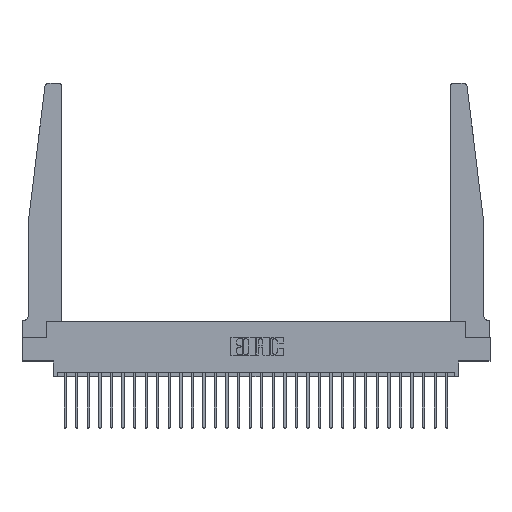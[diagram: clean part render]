
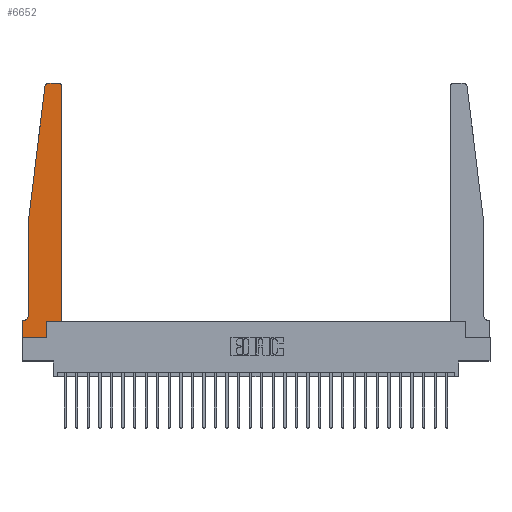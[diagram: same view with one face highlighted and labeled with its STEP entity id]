
A CAD part, top view. The second image highlights one B-rep face of the part: STEP entity #6652.
In plain terms, the highlighted planar face has unit normal (0, 0, 1).
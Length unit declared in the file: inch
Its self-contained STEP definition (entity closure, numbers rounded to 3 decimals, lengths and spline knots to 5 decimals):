
#420 = DIRECTION ( 'NONE',  ( -1., 0., 0. ) ) ;
#589 = ORIENTED_EDGE ( 'NONE', *, *, #18450, .T. ) ;
#660 = ORIENTED_EDGE ( 'NONE', *, *, #11698, .T. ) ;
#1101 = CARTESIAN_POINT ( 'NONE',  ( 0.065, 1.25, 0.37 ) ) ;
#1599 = VECTOR ( 'NONE', #24803, 39.37008 ) ;
#1626 = DIRECTION ( 'NONE',  ( 1., 0., 0. ) ) ;
#1912 = VECTOR ( 'NONE', #25168, 39.37008 ) ;
#2360 = CARTESIAN_POINT ( 'NONE',  ( 0.425, 2.72, 0.37 ) ) ;
#3061 = VECTOR ( 'NONE', #420, 39.37008 ) ;
#3380 = VERTEX_POINT ( 'NONE', #21767 ) ;
#3493 = VERTEX_POINT ( 'NONE', #7417 ) ;
#3578 = DIRECTION ( 'NONE',  ( 0., -1., 0. ) ) ;
#3812 = CARTESIAN_POINT ( 'NONE',  ( 0.425, 0.18, 0.37 ) ) ;
#4221 = EDGE_CURVE ( 'NONE', #23214, #11561, #27533, .T. ) ;
#4247 = PLANE ( 'NONE',  #16551 ) ;
#4533 = DIRECTION ( 'NONE',  ( 1., 0., 0. ) ) ;
#4742 = VERTEX_POINT ( 'NONE', #24952 ) ;
#4785 = LINE ( 'NONE', #15782, #3061 ) ;
#5272 = EDGE_CURVE ( 'NONE', #11561, #4742, #4785, .T. ) ;
#5549 = VERTEX_POINT ( 'NONE', #13014 ) ;
#5551 = ORIENTED_EDGE ( 'NONE', *, *, #10188, .T. ) ;
#5682 = ORIENTED_EDGE ( 'NONE', *, *, #17582, .T. ) ;
#5977 = CIRCLE ( 'NONE', #16139, 0.03 ) ;
#6006 = LINE ( 'NONE', #3812, #21439 ) ;
#6238 = ORIENTED_EDGE ( 'NONE', *, *, #13236, .T. ) ;
#6507 = ORIENTED_EDGE ( 'NONE', *, *, #4221, .T. ) ;
#6628 = LINE ( 'NONE', #8801, #23056 ) ;
#6652 = ADVANCED_FACE ( 'NONE', ( #22059 ), #4247, .T. ) ;
#7417 = CARTESIAN_POINT ( 'NONE',  ( 0.2605, 0., 0.37 ) ) ;
#7433 = LINE ( 'NONE', #9739, #26923 ) ;
#7542 = EDGE_CURVE ( 'NONE', #23935, #24963, #20275, .T. ) ;
#8082 = CARTESIAN_POINT ( 'NONE',  ( 0.27653, 2.72, 0.37 ) ) ;
#8221 = ORIENTED_EDGE ( 'NONE', *, *, #17091, .T. ) ;
#8432 = DIRECTION ( 'NONE',  ( 0., -1., 0. ) ) ;
#8518 = DIRECTION ( 'NONE',  ( 0., 1., 0. ) ) ;
#8801 = CARTESIAN_POINT ( 'NONE',  ( 0.425, 0.18, 0.37 ) ) ;
#8932 = DIRECTION ( 'NONE',  ( -1., 0., 0. ) ) ;
#8957 = EDGE_LOOP ( 'NONE', ( #25474, #589, #660, #5682, #6507, #20017, #25842, #22863, #8221, #6238, #5551, #11950 ) ) ;
#9621 = CARTESIAN_POINT ( 'NONE',  ( 0., 0., 0.37 ) ) ;
#9739 = CARTESIAN_POINT ( 'NONE',  ( 0.25, 2.75, 0.37 ) ) ;
#10188 = EDGE_CURVE ( 'NONE', #20077, #23935, #6628, .T. ) ;
#10887 = DIRECTION ( 'NONE',  ( 0., 0., 1. ) ) ;
#11086 = DIRECTION ( 'NONE',  ( 0., 0., 1. ) ) ;
#11533 = CARTESIAN_POINT ( 'NONE',  ( 0.395, 2.75, 0.37 ) ) ;
#11554 = CARTESIAN_POINT ( 'NONE',  ( 0.015, 0.2375, 0.37 ) ) ;
#11561 = VERTEX_POINT ( 'NONE', #13608 ) ;
#11634 = DIRECTION ( 'NONE',  ( -1., 0., 0. ) ) ;
#11698 = EDGE_CURVE ( 'NONE', #15512, #12809, #18661, .T. ) ;
#11847 = CARTESIAN_POINT ( 'NONE',  ( 0.065, 1.25, 0.37 ) ) ;
#11950 = ORIENTED_EDGE ( 'NONE', *, *, #7542, .T. ) ;
#12274 = CARTESIAN_POINT ( 'NONE',  ( 0.24675, 2.72367, 0.37 ) ) ;
#12420 = EDGE_CURVE ( 'NONE', #24963, #3380, #7433, .T. ) ;
#12809 = VERTEX_POINT ( 'NONE', #11847 ) ;
#13014 = CARTESIAN_POINT ( 'NONE',  ( 0.2605, 0.18, 0.37 ) ) ;
#13236 = EDGE_CURVE ( 'NONE', #5549, #20077, #6006, .T. ) ;
#13608 = CARTESIAN_POINT ( 'NONE',  ( 0.015, 0.1875, 0.37 ) ) ;
#13748 = CARTESIAN_POINT ( 'NONE',  ( 0.065, 0.2375, 0.37 ) ) ;
#13942 = VERTEX_POINT ( 'NONE', #22431 ) ;
#14589 = LINE ( 'NONE', #16933, #15014 ) ;
#15014 = VECTOR ( 'NONE', #3578, 39.37008 ) ;
#15512 = VERTEX_POINT ( 'NONE', #12274 ) ;
#15782 = CARTESIAN_POINT ( 'NONE',  ( 0.065, 0.1875, 0.37 ) ) ;
#16139 = AXIS2_PLACEMENT_3D ( 'NONE', #8082, #25747, #28357 ) ;
#16161 = LINE ( 'NONE', #9621, #23203 ) ;
#16551 = AXIS2_PLACEMENT_3D ( 'NONE', #19752, #10887, #4533 ) ;
#16601 = EDGE_CURVE ( 'NONE', #4742, #13942, #14589, .T. ) ;
#16615 = CARTESIAN_POINT ( 'NONE',  ( 0.2605, 0.18, 0.37 ) ) ;
#16933 = CARTESIAN_POINT ( 'NONE',  ( 0., 0., 0.37 ) ) ;
#17091 = EDGE_CURVE ( 'NONE', #3493, #5549, #21227, .T. ) ;
#17291 = LINE ( 'NONE', #22046, #21331 ) ;
#17582 = EDGE_CURVE ( 'NONE', #12809, #23214, #17291, .T. ) ;
#18450 = EDGE_CURVE ( 'NONE', #3380, #15512, #5977, .T. ) ;
#18661 = LINE ( 'NONE', #1101, #1912 ) ;
#19752 = CARTESIAN_POINT ( 'NONE',  ( 0., 0.1875, 0.37 ) ) ;
#20017 = ORIENTED_EDGE ( 'NONE', *, *, #5272, .T. ) ;
#20077 = VERTEX_POINT ( 'NONE', #21089 ) ;
#20275 = CIRCLE ( 'NONE', #26738, 0.03 ) ;
#21089 = CARTESIAN_POINT ( 'NONE',  ( 0.425, 0.18, 0.37 ) ) ;
#21227 = LINE ( 'NONE', #16615, #1599 ) ;
#21331 = VECTOR ( 'NONE', #8432, 39.37008 ) ;
#21439 = VECTOR ( 'NONE', #1626, 39.37008 ) ;
#21512 = AXIS2_PLACEMENT_3D ( 'NONE', #11554, #22423, #8932 ) ;
#21767 = CARTESIAN_POINT ( 'NONE',  ( 0.27653, 2.75, 0.37 ) ) ;
#22046 = CARTESIAN_POINT ( 'NONE',  ( 0.065, 1.25, 0.37 ) ) ;
#22059 = FACE_OUTER_BOUND ( 'NONE', #8957, .T. ) ;
#22250 = CARTESIAN_POINT ( 'NONE',  ( 0.395, 2.72, 0.37 ) ) ;
#22269 = EDGE_CURVE ( 'NONE', #13942, #3493, #16161, .T. ) ;
#22423 = DIRECTION ( 'NONE',  ( 0., 0., -1. ) ) ;
#22431 = CARTESIAN_POINT ( 'NONE',  ( 0., 0., 0.37 ) ) ;
#22680 = DIRECTION ( 'NONE',  ( 1., 0., 0. ) ) ;
#22863 = ORIENTED_EDGE ( 'NONE', *, *, #22269, .T. ) ;
#23056 = VECTOR ( 'NONE', #8518, 39.37008 ) ;
#23203 = VECTOR ( 'NONE', #22680, 39.37008 ) ;
#23214 = VERTEX_POINT ( 'NONE', #13748 ) ;
#23935 = VERTEX_POINT ( 'NONE', #2360 ) ;
#24555 = DIRECTION ( 'NONE',  ( 1., 0., 0. ) ) ;
#24803 = DIRECTION ( 'NONE',  ( 0., 1., 0. ) ) ;
#24952 = CARTESIAN_POINT ( 'NONE',  ( 0., 0.1875, 0.37 ) ) ;
#24963 = VERTEX_POINT ( 'NONE', #11533 ) ;
#25168 = DIRECTION ( 'NONE',  ( -0.122, -0.992, 0. ) ) ;
#25474 = ORIENTED_EDGE ( 'NONE', *, *, #12420, .T. ) ;
#25747 = DIRECTION ( 'NONE',  ( 0., 0., 1. ) ) ;
#25842 = ORIENTED_EDGE ( 'NONE', *, *, #16601, .T. ) ;
#26738 = AXIS2_PLACEMENT_3D ( 'NONE', #22250, #11086, #24555 ) ;
#26923 = VECTOR ( 'NONE', #11634, 39.37008 ) ;
#27533 = CIRCLE ( 'NONE', #21512, 0.05 ) ;
#28357 = DIRECTION ( 'NONE',  ( 1., 0., 0. ) ) ;
